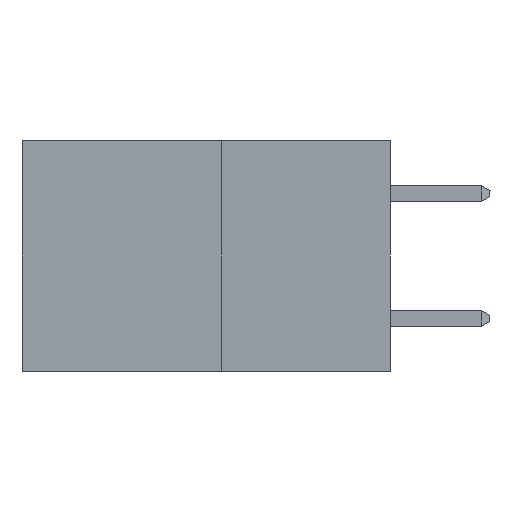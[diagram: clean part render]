
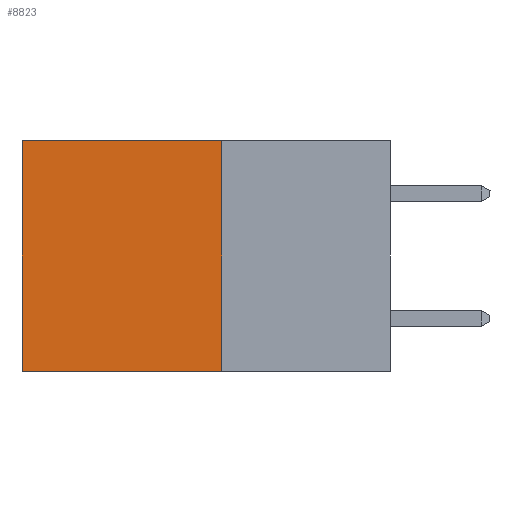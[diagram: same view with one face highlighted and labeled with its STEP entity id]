
A CAD part, left-side view. The second image highlights one B-rep face of the part: STEP entity #8823.
In plain terms, the highlighted planar face has unit normal (-1, 0, 0).
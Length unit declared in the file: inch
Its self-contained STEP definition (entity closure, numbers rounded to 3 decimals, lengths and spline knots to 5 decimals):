
#156 = EDGE_CURVE ( 'NONE', #353, #2102, #1332, .T. ) ;
#353 = VERTEX_POINT ( 'NONE', #4874 ) ;
#382 = DIRECTION ( 'NONE',  ( 1., 0., 0. ) ) ;
#678 = DIRECTION ( 'NONE',  ( 0., 1., 0. ) ) ;
#1332 = LINE ( 'NONE', #4973, #7586 ) ;
#1362 = VERTEX_POINT ( 'NONE', #7507 ) ;
#1387 = VECTOR ( 'NONE', #5799, 39.37008 ) ;
#1476 = ORIENTED_EDGE ( 'NONE', *, *, #156, .T. ) ;
#1716 = ORIENTED_EDGE ( 'NONE', *, *, #9686, .T. ) ;
#2044 = VECTOR ( 'NONE', #2260, 39.37008 ) ;
#2102 = VERTEX_POINT ( 'NONE', #5289 ) ;
#2260 = DIRECTION ( 'NONE',  ( 0., 1., 0. ) ) ;
#4874 = CARTESIAN_POINT ( 'NONE',  ( 0.277, 0.59, 0. ) ) ;
#4973 = CARTESIAN_POINT ( 'NONE',  ( 0.277, 0.59, -0.37 ) ) ;
#5289 = CARTESIAN_POINT ( 'NONE',  ( 0.277, 0.59, -0.37 ) ) ;
#5425 = CARTESIAN_POINT ( 'NONE',  ( 0.277, 0.27, -0.37 ) ) ;
#5724 = DIRECTION ( 'NONE',  ( 0., 0., -1. ) ) ;
#5799 = DIRECTION ( 'NONE',  ( 0., 0., -1. ) ) ;
#5920 = DIRECTION ( 'NONE',  ( 0., 0., -1. ) ) ;
#6168 = CARTESIAN_POINT ( 'NONE',  ( 0.277, 0.27, -0.37 ) ) ;
#6197 = CARTESIAN_POINT ( 'NONE',  ( 0.277, 0.27, 0. ) ) ;
#6247 = FACE_OUTER_BOUND ( 'NONE', #9786, .T. ) ;
#7229 = EDGE_CURVE ( 'NONE', #1362, #8439, #9074, .T. ) ;
#7401 = CARTESIAN_POINT ( 'NONE',  ( 0.277, 0.27, -0.37 ) ) ;
#7507 = CARTESIAN_POINT ( 'NONE',  ( 0.277, 0.27, 0. ) ) ;
#7586 = VECTOR ( 'NONE', #5724, 39.37008 ) ;
#7664 = ORIENTED_EDGE ( 'NONE', *, *, #9658, .F. ) ;
#7678 = VECTOR ( 'NONE', #678, 39.37008 ) ;
#8439 = VERTEX_POINT ( 'NONE', #5425 ) ;
#8823 = ADVANCED_FACE ( 'NONE', ( #6247 ), #8885, .F. ) ;
#8885 = PLANE ( 'NONE',  #8977 ) ;
#8977 = AXIS2_PLACEMENT_3D ( 'NONE', #7401, #382, #5920 ) ;
#9074 = LINE ( 'NONE', #9502, #1387 ) ;
#9448 = LINE ( 'NONE', #6197, #7678 ) ;
#9502 = CARTESIAN_POINT ( 'NONE',  ( 0.277, 0.27, -0.37 ) ) ;
#9609 = ORIENTED_EDGE ( 'NONE', *, *, #7229, .F. ) ;
#9658 = EDGE_CURVE ( 'NONE', #8439, #2102, #9716, .T. ) ;
#9686 = EDGE_CURVE ( 'NONE', #1362, #353, #9448, .T. ) ;
#9716 = LINE ( 'NONE', #6168, #2044 ) ;
#9786 = EDGE_LOOP ( 'NONE', ( #1476, #7664, #9609, #1716 ) ) ;
